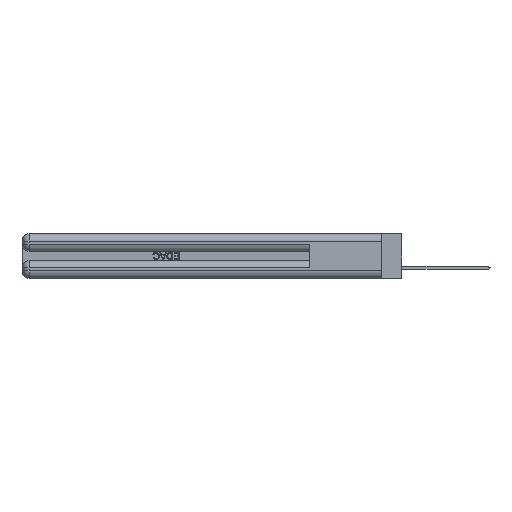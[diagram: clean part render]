
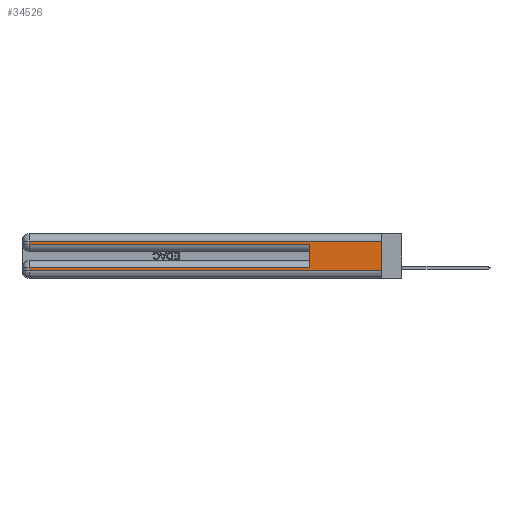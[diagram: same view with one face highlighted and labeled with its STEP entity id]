
A CAD part, left-side view. The second image highlights one B-rep face of the part: STEP entity #34526.
In plain terms, the highlighted planar face has unit normal (-1, 0, 0).
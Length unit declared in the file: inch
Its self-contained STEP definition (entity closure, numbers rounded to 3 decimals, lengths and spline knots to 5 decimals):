
#409 = DIRECTION ( 'NONE',  ( 0., 1., 0. ) ) ;
#1144 = FACE_OUTER_BOUND ( 'NONE', #40746, .T. ) ;
#2650 = ORIENTED_EDGE ( 'NONE', *, *, #36579, .T. ) ;
#2659 = ORIENTED_EDGE ( 'NONE', *, *, #24870, .T. ) ;
#3041 = CARTESIAN_POINT ( 'NONE',  ( 0., 0., 0.31 ) ) ;
#3727 = CARTESIAN_POINT ( 'NONE',  ( 0., 0., 0.06 ) ) ;
#4333 = ORIENTED_EDGE ( 'NONE', *, *, #18660, .T. ) ;
#5138 = LINE ( 'NONE', #12244, #20948 ) ;
#5670 = CARTESIAN_POINT ( 'NONE',  ( 0., 0., 0.37 ) ) ;
#6370 = DIRECTION ( 'NONE',  ( 0., 0., 1. ) ) ;
#6452 = CARTESIAN_POINT ( 'NONE',  ( 0., 0., 0.37 ) ) ;
#8168 = EDGE_CURVE ( 'NONE', #17996, #15111, #36435, .T. ) ;
#8190 = CARTESIAN_POINT ( 'NONE',  ( 0., 2.94, 0.085 ) ) ;
#8941 = CARTESIAN_POINT ( 'NONE',  ( 0., 0., 0.285 ) ) ;
#8986 = DIRECTION ( 'NONE',  ( 0., 0., -1. ) ) ;
#10771 = CARTESIAN_POINT ( 'NONE',  ( 0., 0.6, 0.085 ) ) ;
#12244 = CARTESIAN_POINT ( 'NONE',  ( 0., 0., 0.085 ) ) ;
#13543 = EDGE_CURVE ( 'NONE', #15111, #22210, #33529, .T. ) ;
#15111 = VERTEX_POINT ( 'NONE', #16849 ) ;
#15789 = VERTEX_POINT ( 'NONE', #10771 ) ;
#15882 = VERTEX_POINT ( 'NONE', #8190 ) ;
#16134 = CARTESIAN_POINT ( 'NONE',  ( 0., 0.6, 0.145 ) ) ;
#16849 = CARTESIAN_POINT ( 'NONE',  ( 0., 2.94, 0.31 ) ) ;
#16912 = DIRECTION ( 'NONE',  ( 0., -1., 0. ) ) ;
#17996 = VERTEX_POINT ( 'NONE', #3041 ) ;
#18520 = ORIENTED_EDGE ( 'NONE', *, *, #27670, .F. ) ;
#18660 = EDGE_CURVE ( 'NONE', #15882, #32649, #39287, .T. ) ;
#18971 = DIRECTION ( 'NONE',  ( 0., -1., 0. ) ) ;
#19227 = DIRECTION ( 'NONE',  ( 1., 0., 0. ) ) ;
#20801 = CARTESIAN_POINT ( 'NONE',  ( 0., 2.94, 0.285 ) ) ;
#20948 = VECTOR ( 'NONE', #31292, 39.37008 ) ;
#21835 = DIRECTION ( 'NONE',  ( 0., 0., -1. ) ) ;
#22210 = VERTEX_POINT ( 'NONE', #20801 ) ;
#22715 = CARTESIAN_POINT ( 'NONE',  ( 0., 2.94, 0.37 ) ) ;
#23906 = AXIS2_PLACEMENT_3D ( 'NONE', #6452, #19227, #25646 ) ;
#24870 = EDGE_CURVE ( 'NONE', #32649, #32519, #42360, .T. ) ;
#25126 = VERTEX_POINT ( 'NONE', #37269 ) ;
#25427 = CARTESIAN_POINT ( 'NONE',  ( 0., 2.94, 0.37 ) ) ;
#25646 = DIRECTION ( 'NONE',  ( 0., 0., -1. ) ) ;
#25973 = VECTOR ( 'NONE', #18971, 39.37008 ) ;
#27032 = ORIENTED_EDGE ( 'NONE', *, *, #8168, .T. ) ;
#27670 = EDGE_CURVE ( 'NONE', #17996, #32519, #31581, .T. ) ;
#28027 = LINE ( 'NONE', #16134, #41423 ) ;
#28259 = CARTESIAN_POINT ( 'NONE',  ( 0., 2.94, 0.06 ) ) ;
#28818 = PLANE ( 'NONE',  #23906 ) ;
#29378 = ORIENTED_EDGE ( 'NONE', *, *, #13543, .T. ) ;
#29484 = VECTOR ( 'NONE', #35921, 39.37008 ) ;
#29754 = VECTOR ( 'NONE', #409, 39.37008 ) ;
#31292 = DIRECTION ( 'NONE',  ( 0., 1., 0. ) ) ;
#31581 = LINE ( 'NONE', #5670, #35687 ) ;
#32519 = VERTEX_POINT ( 'NONE', #40193 ) ;
#32604 = ORIENTED_EDGE ( 'NONE', *, *, #39452, .F. ) ;
#32649 = VERTEX_POINT ( 'NONE', #28259 ) ;
#33526 = VECTOR ( 'NONE', #16912, 39.37008 ) ;
#33529 = LINE ( 'NONE', #25427, #39230 ) ;
#34526 = ADVANCED_FACE ( 'NONE', ( #1144 ), #28818, .F. ) ;
#34730 = LINE ( 'NONE', #8941, #25973 ) ;
#35687 = VECTOR ( 'NONE', #21835, 39.37008 ) ;
#35921 = DIRECTION ( 'NONE',  ( 0., 0., -1. ) ) ;
#36435 = LINE ( 'NONE', #39257, #29754 ) ;
#36579 = EDGE_CURVE ( 'NONE', #15789, #15882, #5138, .T. ) ;
#37269 = CARTESIAN_POINT ( 'NONE',  ( 0., 0.6, 0.285 ) ) ;
#38052 = EDGE_CURVE ( 'NONE', #22210, #25126, #34730, .T. ) ;
#39217 = ORIENTED_EDGE ( 'NONE', *, *, #38052, .T. ) ;
#39230 = VECTOR ( 'NONE', #8986, 39.37008 ) ;
#39257 = CARTESIAN_POINT ( 'NONE',  ( 0., 0., 0.31 ) ) ;
#39287 = LINE ( 'NONE', #22715, #29484 ) ;
#39452 = EDGE_CURVE ( 'NONE', #15789, #25126, #28027, .T. ) ;
#40193 = CARTESIAN_POINT ( 'NONE',  ( 0., 0., 0.06 ) ) ;
#40746 = EDGE_LOOP ( 'NONE', ( #18520, #27032, #29378, #39217, #32604, #2650, #4333, #2659 ) ) ;
#41423 = VECTOR ( 'NONE', #6370, 39.37008 ) ;
#42360 = LINE ( 'NONE', #3727, #33526 ) ;
